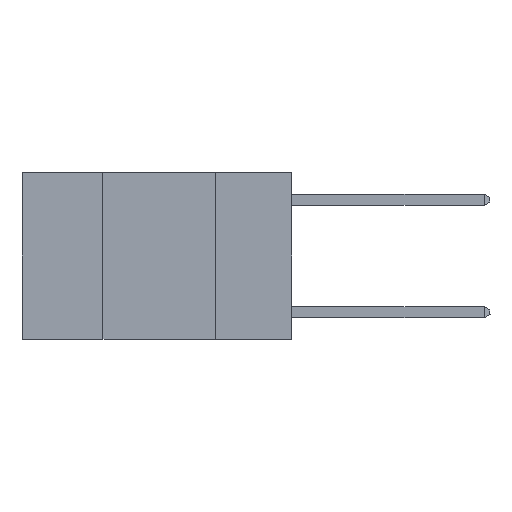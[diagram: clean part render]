
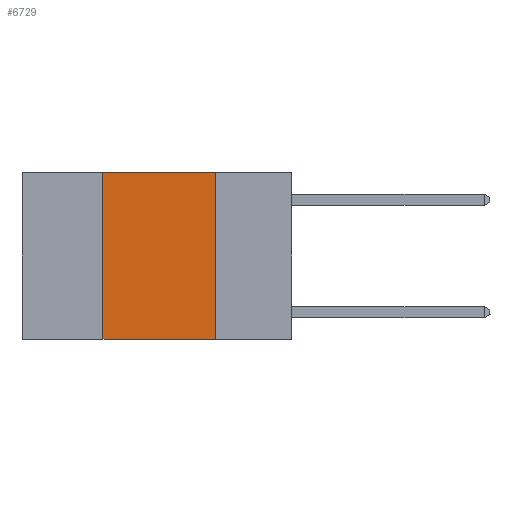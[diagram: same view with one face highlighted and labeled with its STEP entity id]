
A CAD part, left-side view. The second image highlights one B-rep face of the part: STEP entity #6729.
In plain terms, the highlighted planar face has unit normal (-1, 0, 0).
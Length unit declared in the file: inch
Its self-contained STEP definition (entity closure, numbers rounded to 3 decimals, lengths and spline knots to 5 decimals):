
#239 = DIRECTION ( 'NONE',  ( 0., -1., 0. ) ) ;
#532 = VERTEX_POINT ( 'NONE', #4482 ) ;
#776 = VECTOR ( 'NONE', #16498, 39.37008 ) ;
#1026 = EDGE_CURVE ( 'NONE', #3929, #9837, #11077, .T. ) ;
#3318 = LINE ( 'NONE', #14874, #22318 ) ;
#3713 = VECTOR ( 'NONE', #19319, 39.37008 ) ;
#3831 = VECTOR ( 'NONE', #239, 39.37008 ) ;
#3929 = VERTEX_POINT ( 'NONE', #19309 ) ;
#4039 = CARTESIAN_POINT ( 'NONE',  ( 0., 0.6, -0.37 ) ) ;
#4311 = LINE ( 'NONE', #4039, #3713 ) ;
#4482 = CARTESIAN_POINT ( 'NONE',  ( 0., 0.17, -0.37 ) ) ;
#5106 = DIRECTION ( 'NONE',  ( 0., 0., -1. ) ) ;
#6729 = ADVANCED_FACE ( 'NONE', ( #22247 ), #14686, .F. ) ;
#7101 = EDGE_CURVE ( 'NONE', #9837, #10325, #23830, .T. ) ;
#7709 = ORIENTED_EDGE ( 'NONE', *, *, #14361, .T. ) ;
#8045 = ORIENTED_EDGE ( 'NONE', *, *, #1026, .F. ) ;
#8389 = ORIENTED_EDGE ( 'NONE', *, *, #7101, .F. ) ;
#8490 = ORIENTED_EDGE ( 'NONE', *, *, #23106, .F. ) ;
#9837 = VERTEX_POINT ( 'NONE', #18753 ) ;
#10325 = VERTEX_POINT ( 'NONE', #23377 ) ;
#11077 = LINE ( 'NONE', #23730, #776 ) ;
#11534 = EDGE_LOOP ( 'NONE', ( #8490, #8389, #8045, #7709 ) ) ;
#12751 = CARTESIAN_POINT ( 'NONE',  ( 0., 0.6, 0. ) ) ;
#14361 = EDGE_CURVE ( 'NONE', #3929, #532, #4311, .T. ) ;
#14686 = PLANE ( 'NONE',  #19066 ) ;
#14874 = CARTESIAN_POINT ( 'NONE',  ( 0., 0.17, 0. ) ) ;
#14961 = DIRECTION ( 'NONE',  ( 0., 0., -1. ) ) ;
#16498 = DIRECTION ( 'NONE',  ( 0., 0., 1. ) ) ;
#16619 = DIRECTION ( 'NONE',  ( 1., 0., 0. ) ) ;
#18753 = CARTESIAN_POINT ( 'NONE',  ( 0., 0.42, 0. ) ) ;
#19066 = AXIS2_PLACEMENT_3D ( 'NONE', #12751, #16619, #5106 ) ;
#19309 = CARTESIAN_POINT ( 'NONE',  ( 0., 0.42, -0.37 ) ) ;
#19319 = DIRECTION ( 'NONE',  ( 0., -1., 0. ) ) ;
#19533 = CARTESIAN_POINT ( 'NONE',  ( 0., 0.6, 0. ) ) ;
#22247 = FACE_OUTER_BOUND ( 'NONE', #11534, .T. ) ;
#22318 = VECTOR ( 'NONE', #14961, 39.37008 ) ;
#23106 = EDGE_CURVE ( 'NONE', #10325, #532, #3318, .T. ) ;
#23377 = CARTESIAN_POINT ( 'NONE',  ( 0., 0.17, 0. ) ) ;
#23730 = CARTESIAN_POINT ( 'NONE',  ( 0., 0.42, 0. ) ) ;
#23830 = LINE ( 'NONE', #19533, #3831 ) ;
